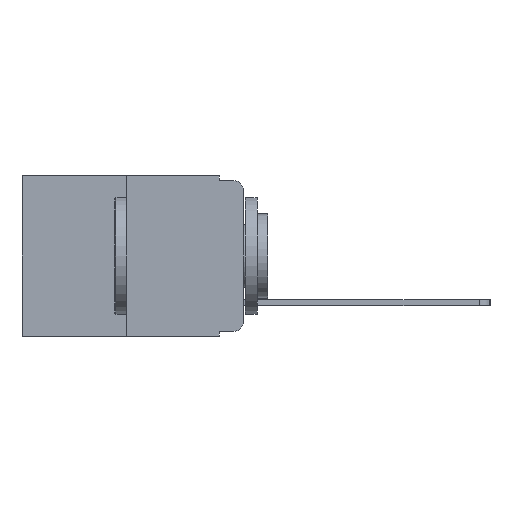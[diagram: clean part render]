
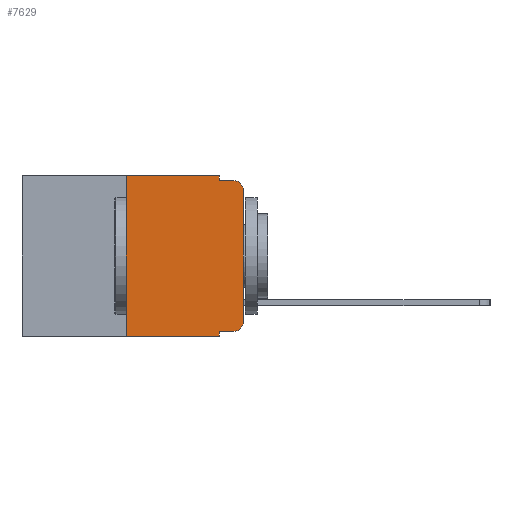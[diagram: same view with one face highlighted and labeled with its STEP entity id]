
A CAD part, left-side view. The second image highlights one B-rep face of the part: STEP entity #7629.
In plain terms, the highlighted planar face has unit normal (-1, 0, 0).
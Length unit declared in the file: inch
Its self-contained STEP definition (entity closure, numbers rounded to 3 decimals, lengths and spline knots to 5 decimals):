
#160 = VERTEX_POINT ( 'NONE', #20430 ) ;
#800 = LINE ( 'NONE', #7914, #3955 ) ;
#1384 = EDGE_CURVE ( 'NONE', #6272, #160, #6568, .T. ) ;
#1491 = VERTEX_POINT ( 'NONE', #9924 ) ;
#1701 = ORIENTED_EDGE ( 'NONE', *, *, #3633, .T. ) ;
#1934 = VECTOR ( 'NONE', #9632, 39.37008 ) ;
#2117 = VERTEX_POINT ( 'NONE', #16434 ) ;
#2570 = DIRECTION ( 'NONE',  ( -1., 0., 0. ) ) ;
#2889 = CARTESIAN_POINT ( 'NONE',  ( 0., 0.25, 0. ) ) ;
#3040 = EDGE_CURVE ( 'NONE', #5569, #8928, #21387, .T. ) ;
#3503 = VERTEX_POINT ( 'NONE', #20324 ) ;
#3633 = EDGE_CURVE ( 'NONE', #160, #8928, #6459, .T. ) ;
#3851 = ORIENTED_EDGE ( 'NONE', *, *, #19343, .T. ) ;
#3917 = DIRECTION ( 'NONE',  ( 0., 0., -1. ) ) ;
#3955 = VECTOR ( 'NONE', #6306, 39.37008 ) ;
#4347 = CARTESIAN_POINT ( 'NONE',  ( 0., 0.473, 0. ) ) ;
#4560 = VECTOR ( 'NONE', #18916, 39.37008 ) ;
#5246 = VECTOR ( 'NONE', #9183, 39.37008 ) ;
#5569 = VERTEX_POINT ( 'NONE', #6133 ) ;
#5937 = LINE ( 'NONE', #11910, #18401 ) ;
#6053 = CARTESIAN_POINT ( 'NONE',  ( 0., 0.051, -0.333 ) ) ;
#6103 = DIRECTION ( 'NONE',  ( 0., 0., -1. ) ) ;
#6133 = CARTESIAN_POINT ( 'NONE',  ( 0., 0.051, -0.01 ) ) ;
#6272 = VERTEX_POINT ( 'NONE', #17929 ) ;
#6306 = DIRECTION ( 'NONE',  ( 0., -1., 0. ) ) ;
#6459 = CIRCLE ( 'NONE', #10833, 0.02 ) ;
#6568 = LINE ( 'NONE', #7970, #1934 ) ;
#6866 = ORIENTED_EDGE ( 'NONE', *, *, #3040, .F. ) ;
#6879 = AXIS2_PLACEMENT_3D ( 'NONE', #7867, #19162, #9533 ) ;
#7515 = CARTESIAN_POINT ( 'NONE',  ( 0., 0.051, 0. ) ) ;
#7629 = ADVANCED_FACE ( 'NONE', ( #16042 ), #14377, .F. ) ;
#7867 = CARTESIAN_POINT ( 'NONE',  ( 0., 0.02, -0.313 ) ) ;
#7888 = ORIENTED_EDGE ( 'NONE', *, *, #14858, .F. ) ;
#7914 = CARTESIAN_POINT ( 'NONE',  ( 0., 0.473, 0. ) ) ;
#7970 = CARTESIAN_POINT ( 'NONE',  ( 0., 0., 0. ) ) ;
#8195 = CARTESIAN_POINT ( 'NONE',  ( 0., 0.02, -0.01 ) ) ;
#8928 = VERTEX_POINT ( 'NONE', #8195 ) ;
#9183 = DIRECTION ( 'NONE',  ( 0., 0., -1. ) ) ;
#9288 = CARTESIAN_POINT ( 'NONE',  ( 0., 0.051, -0.01 ) ) ;
#9457 = ORIENTED_EDGE ( 'NONE', *, *, #10403, .T. ) ;
#9533 = DIRECTION ( 'NONE',  ( 0., 0., -1. ) ) ;
#9632 = DIRECTION ( 'NONE',  ( 0., 0., 1. ) ) ;
#9635 = DIRECTION ( 'NONE',  ( 0., 0., 1. ) ) ;
#9725 = CARTESIAN_POINT ( 'NONE',  ( 0., 0.051, 0. ) ) ;
#9924 = CARTESIAN_POINT ( 'NONE',  ( 0., 0.051, -0.333 ) ) ;
#10170 = VERTEX_POINT ( 'NONE', #12280 ) ;
#10403 = EDGE_CURVE ( 'NONE', #11834, #6272, #13241, .T. ) ;
#10742 = CARTESIAN_POINT ( 'NONE',  ( 0., 0.051, 0. ) ) ;
#10833 = AXIS2_PLACEMENT_3D ( 'NONE', #12752, #2570, #14349 ) ;
#11475 = LINE ( 'NONE', #6053, #19946 ) ;
#11544 = EDGE_CURVE ( 'NONE', #1491, #11834, #11475, .T. ) ;
#11834 = VERTEX_POINT ( 'NONE', #21271 ) ;
#11910 = CARTESIAN_POINT ( 'NONE',  ( 0., 0.473, -0.343 ) ) ;
#12280 = CARTESIAN_POINT ( 'NONE',  ( 0., 0.25, 0. ) ) ;
#12752 = CARTESIAN_POINT ( 'NONE',  ( 0., 0.02, -0.03 ) ) ;
#13241 = CIRCLE ( 'NONE', #6879, 0.02 ) ;
#13840 = VECTOR ( 'NONE', #9635, 39.37008 ) ;
#14349 = DIRECTION ( 'NONE',  ( 0., 0., -1. ) ) ;
#14377 = PLANE ( 'NONE',  #15392 ) ;
#14605 = ORIENTED_EDGE ( 'NONE', *, *, #1384, .T. ) ;
#14858 = EDGE_CURVE ( 'NONE', #2117, #10170, #18014, .T. ) ;
#15392 = AXIS2_PLACEMENT_3D ( 'NONE', #4347, #15949, #6103 ) ;
#15596 = ORIENTED_EDGE ( 'NONE', *, *, #20618, .F. ) ;
#15909 = DIRECTION ( 'NONE',  ( 0., -1., 0. ) ) ;
#15949 = DIRECTION ( 'NONE',  ( 1., 0., 0. ) ) ;
#16042 = FACE_OUTER_BOUND ( 'NONE', #17641, .T. ) ;
#16080 = ORIENTED_EDGE ( 'NONE', *, *, #16450, .F. ) ;
#16434 = CARTESIAN_POINT ( 'NONE',  ( 0., 0.25, -0.343 ) ) ;
#16450 = EDGE_CURVE ( 'NONE', #10170, #16495, #800, .T. ) ;
#16495 = VERTEX_POINT ( 'NONE', #9725 ) ;
#17061 = ORIENTED_EDGE ( 'NONE', *, *, #18836, .F. ) ;
#17534 = ORIENTED_EDGE ( 'NONE', *, *, #11544, .T. ) ;
#17641 = EDGE_LOOP ( 'NONE', ( #14605, #1701, #6866, #15596, #16080, #7888, #3851, #17061, #17534, #9457 ) ) ;
#17929 = CARTESIAN_POINT ( 'NONE',  ( 0., 0., -0.313 ) ) ;
#18014 = LINE ( 'NONE', #2889, #13840 ) ;
#18275 = LINE ( 'NONE', #7515, #5246 ) ;
#18401 = VECTOR ( 'NONE', #19805, 39.37008 ) ;
#18836 = EDGE_CURVE ( 'NONE', #1491, #3503, #19952, .T. ) ;
#18916 = DIRECTION ( 'NONE',  ( 0., -1., 0. ) ) ;
#19162 = DIRECTION ( 'NONE',  ( -1., 0., 0. ) ) ;
#19343 = EDGE_CURVE ( 'NONE', #2117, #3503, #5937, .T. ) ;
#19805 = DIRECTION ( 'NONE',  ( 0., -1., 0. ) ) ;
#19946 = VECTOR ( 'NONE', #15909, 39.37008 ) ;
#19952 = LINE ( 'NONE', #10742, #20424 ) ;
#20324 = CARTESIAN_POINT ( 'NONE',  ( 0., 0.051, -0.343 ) ) ;
#20424 = VECTOR ( 'NONE', #3917, 39.37008 ) ;
#20430 = CARTESIAN_POINT ( 'NONE',  ( 0., 0., -0.03 ) ) ;
#20618 = EDGE_CURVE ( 'NONE', #16495, #5569, #18275, .T. ) ;
#21271 = CARTESIAN_POINT ( 'NONE',  ( 0., 0.02, -0.333 ) ) ;
#21387 = LINE ( 'NONE', #9288, #4560 ) ;
